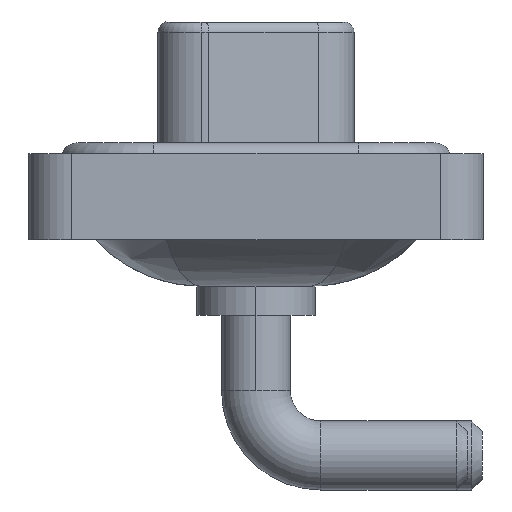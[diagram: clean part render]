
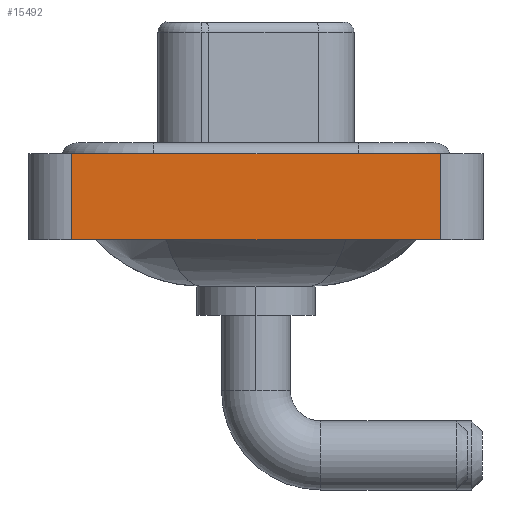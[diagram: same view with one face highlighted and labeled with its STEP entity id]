
A CAD part, left-side view. The second image highlights one B-rep face of the part: STEP entity #15492.
In plain terms, the highlighted planar face has unit normal (-1, 0, 0).
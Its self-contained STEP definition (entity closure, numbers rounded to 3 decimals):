
#249 = DIRECTION ( 'NONE',  ( 0., 0., 1. ) ) ;
#269 = DIRECTION ( 'NONE',  ( 0., 0., 1. ) ) ;
#496 = CARTESIAN_POINT ( 'NONE',  ( -7.3, -8.55, 0.4 ) ) ;
#582 = EDGE_CURVE ( 'NONE', #7208, #17138, #10980, .T. ) ;
#1333 = LINE ( 'NONE', #7013, #16224 ) ;
#1429 = DIRECTION ( 'NONE',  ( 0., -1., 0. ) ) ;
#1629 = CARTESIAN_POINT ( 'NONE',  ( -7.3, -8.55, -3.6 ) ) ;
#1777 = VECTOR ( 'NONE', #6103, 1000. ) ;
#1831 = CARTESIAN_POINT ( 'NONE',  ( -7.3, -8.55, -3.6 ) ) ;
#2256 = VECTOR ( 'NONE', #249, 1000. ) ;
#3405 = DIRECTION ( 'NONE',  ( -1., 0., 0. ) ) ;
#4155 = EDGE_LOOP ( 'NONE', ( #5080, #11143, #8914, #13452 ) ) ;
#4517 = VERTEX_POINT ( 'NONE', #1629 ) ;
#4553 = EDGE_CURVE ( 'NONE', #13538, #7208, #11887, .T. ) ;
#4978 = FACE_OUTER_BOUND ( 'NONE', #4155, .T. ) ;
#5080 = ORIENTED_EDGE ( 'NONE', *, *, #5835, .T. ) ;
#5835 = EDGE_CURVE ( 'NONE', #4517, #17138, #7610, .T. ) ;
#6103 = DIRECTION ( 'NONE',  ( 0., -1., 0. ) ) ;
#6583 = AXIS2_PLACEMENT_3D ( 'NONE', #16726, #3405, #269 ) ;
#7013 = CARTESIAN_POINT ( 'NONE',  ( -7.3, -8.55, -3.6 ) ) ;
#7208 = VERTEX_POINT ( 'NONE', #17989 ) ;
#7610 = LINE ( 'NONE', #1831, #8583 ) ;
#8583 = VECTOR ( 'NONE', #9368, 1000. ) ;
#8914 = ORIENTED_EDGE ( 'NONE', *, *, #4553, .F. ) ;
#9067 = CARTESIAN_POINT ( 'NONE',  ( -7.3, 8.55, -3.6 ) ) ;
#9368 = DIRECTION ( 'NONE',  ( 0., 0., 1. ) ) ;
#10980 = LINE ( 'NONE', #496, #1777 ) ;
#11143 = ORIENTED_EDGE ( 'NONE', *, *, #582, .F. ) ;
#11463 = CARTESIAN_POINT ( 'NONE',  ( -7.3, 8.55, -3.6 ) ) ;
#11887 = LINE ( 'NONE', #9067, #2256 ) ;
#13452 = ORIENTED_EDGE ( 'NONE', *, *, #17220, .T. ) ;
#13538 = VERTEX_POINT ( 'NONE', #11463 ) ;
#15492 = ADVANCED_FACE ( 'NONE', ( #4978 ), #16819, .T. ) ;
#16224 = VECTOR ( 'NONE', #1429, 1000. ) ;
#16726 = CARTESIAN_POINT ( 'NONE',  ( -7.3, -8.55, -3.6 ) ) ;
#16819 = PLANE ( 'NONE',  #6583 ) ;
#17138 = VERTEX_POINT ( 'NONE', #19124 ) ;
#17220 = EDGE_CURVE ( 'NONE', #13538, #4517, #1333, .T. ) ;
#17989 = CARTESIAN_POINT ( 'NONE',  ( -7.3, 8.55, 0.4 ) ) ;
#19124 = CARTESIAN_POINT ( 'NONE',  ( -7.3, -8.55, 0.4 ) ) ;
